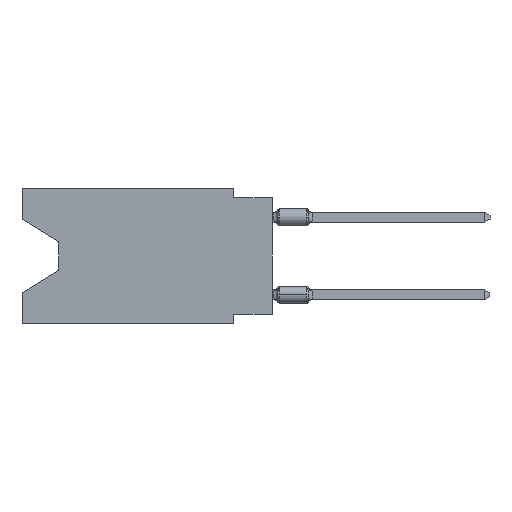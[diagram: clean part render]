
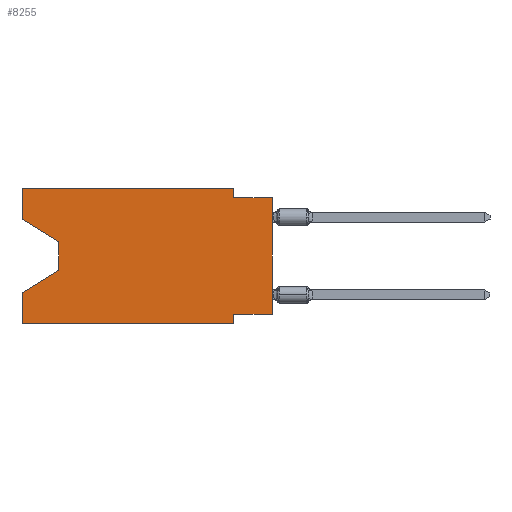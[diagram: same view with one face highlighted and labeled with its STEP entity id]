
A CAD part, left-side view. The second image highlights one B-rep face of the part: STEP entity #8255.
In plain terms, the highlighted planar face has unit normal (-1, 0, 0).
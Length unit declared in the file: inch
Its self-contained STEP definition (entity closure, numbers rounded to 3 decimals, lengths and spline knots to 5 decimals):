
#183 = CARTESIAN_POINT ( 'NONE',  ( 0., 0.645, 0. ) ) ;
#287 = EDGE_CURVE ( 'NONE', #10213, #3877, #16952, .T. ) ;
#308 = CARTESIAN_POINT ( 'NONE',  ( 0., 0.645, 0. ) ) ;
#857 = LINE ( 'NONE', #308, #16641 ) ;
#1285 = DIRECTION ( 'NONE',  ( 0., -1., 0. ) ) ;
#1613 = CARTESIAN_POINT ( 'NONE',  ( 0., 0.55, -0.212 ) ) ;
#1636 = EDGE_CURVE ( 'NONE', #25814, #21088, #18660, .T. ) ;
#1788 = CARTESIAN_POINT ( 'NONE',  ( 0., 0.645, -0.08025 ) ) ;
#1929 = DIRECTION ( 'NONE',  ( 0., -1., 0. ) ) ;
#2426 = DIRECTION ( 'NONE',  ( 0., 0., 1. ) ) ;
#3229 = CARTESIAN_POINT ( 'NONE',  ( 0., 0., -0.325 ) ) ;
#3236 = VECTOR ( 'NONE', #19499, 39.37008 ) ;
#3754 = EDGE_CURVE ( 'NONE', #13657, #24154, #13965, .T. ) ;
#3877 = VERTEX_POINT ( 'NONE', #27752 ) ;
#3882 = PLANE ( 'NONE',  #23036 ) ;
#4906 = EDGE_CURVE ( 'NONE', #6067, #7350, #11999, .T. ) ;
#4974 = DIRECTION ( 'NONE',  ( 0., 0., -1. ) ) ;
#5083 = VECTOR ( 'NONE', #4974, 39.37008 ) ;
#5327 = CARTESIAN_POINT ( 'NONE',  ( 0., 0.645, 0. ) ) ;
#6067 = VERTEX_POINT ( 'NONE', #19371 ) ;
#6144 = ORIENTED_EDGE ( 'NONE', *, *, #21571, .F. ) ;
#6408 = ORIENTED_EDGE ( 'NONE', *, *, #4906, .T. ) ;
#6532 = CARTESIAN_POINT ( 'NONE',  ( 0., 0.645, -0.26975 ) ) ;
#6679 = VECTOR ( 'NONE', #8355, 39.37008 ) ;
#6685 = EDGE_CURVE ( 'NONE', #6067, #21088, #857, .T. ) ;
#6865 = DIRECTION ( 'NONE',  ( 0., 0., 1. ) ) ;
#7350 = VERTEX_POINT ( 'NONE', #10551 ) ;
#8111 = DIRECTION ( 'NONE',  ( 1., 0., 0. ) ) ;
#8255 = ADVANCED_FACE ( 'NONE', ( #20650 ), #3882, .F. ) ;
#8355 = DIRECTION ( 'NONE',  ( 0., 1., 0. ) ) ;
#8492 = DIRECTION ( 'NONE',  ( 0., 0., -1. ) ) ;
#8881 = EDGE_CURVE ( 'NONE', #13657, #10913, #22809, .T. ) ;
#8960 = LINE ( 'NONE', #21652, #16801 ) ;
#9601 = CARTESIAN_POINT ( 'NONE',  ( 0., 0.645, -0.08025 ) ) ;
#10175 = CARTESIAN_POINT ( 'NONE',  ( 0., 0., -0.325 ) ) ;
#10199 = DIRECTION ( 'NONE',  ( 0., 0.855, -0.519 ) ) ;
#10213 = VERTEX_POINT ( 'NONE', #22694 ) ;
#10222 = CARTESIAN_POINT ( 'NONE',  ( 0., 0.645, 0. ) ) ;
#10230 = ORIENTED_EDGE ( 'NONE', *, *, #27822, .F. ) ;
#10551 = CARTESIAN_POINT ( 'NONE',  ( 0., 0.1, -0.35 ) ) ;
#10596 = ORIENTED_EDGE ( 'NONE', *, *, #13782, .T. ) ;
#10913 = VERTEX_POINT ( 'NONE', #17438 ) ;
#11261 = EDGE_CURVE ( 'NONE', #24154, #25814, #19210, .T. ) ;
#11999 = LINE ( 'NONE', #16370, #15288 ) ;
#12247 = VECTOR ( 'NONE', #26757, 39.37008 ) ;
#12577 = CARTESIAN_POINT ( 'NONE',  ( 0., 0.1, 0. ) ) ;
#13657 = VERTEX_POINT ( 'NONE', #1788 ) ;
#13782 = EDGE_CURVE ( 'NONE', #16031, #18413, #8960, .T. ) ;
#13953 = CARTESIAN_POINT ( 'NONE',  ( 0., 0.1, -0.325 ) ) ;
#13965 = LINE ( 'NONE', #9601, #26062 ) ;
#14239 = ORIENTED_EDGE ( 'NONE', *, *, #27090, .F. ) ;
#14951 = VECTOR ( 'NONE', #8492, 39.37008 ) ;
#15288 = VECTOR ( 'NONE', #1285, 39.37008 ) ;
#15967 = ORIENTED_EDGE ( 'NONE', *, *, #287, .F. ) ;
#16031 = VERTEX_POINT ( 'NONE', #3229 ) ;
#16094 = DIRECTION ( 'NONE',  ( 0., -0.855, -0.519 ) ) ;
#16370 = CARTESIAN_POINT ( 'NONE',  ( 0., 0.645, -0.35 ) ) ;
#16641 = VECTOR ( 'NONE', #2426, 39.37008 ) ;
#16756 = CARTESIAN_POINT ( 'NONE',  ( 0., 0.55, -0.138 ) ) ;
#16801 = VECTOR ( 'NONE', #6865, 39.37008 ) ;
#16952 = LINE ( 'NONE', #12577, #19095 ) ;
#17114 = EDGE_CURVE ( 'NONE', #10913, #10213, #23853, .T. ) ;
#17438 = CARTESIAN_POINT ( 'NONE',  ( 0., 0.645, 0. ) ) ;
#17806 = LINE ( 'NONE', #24274, #5083 ) ;
#18413 = VERTEX_POINT ( 'NONE', #23126 ) ;
#18660 = LINE ( 'NONE', #1613, #22263 ) ;
#19095 = VECTOR ( 'NONE', #27387, 39.37008 ) ;
#19210 = LINE ( 'NONE', #27151, #14951 ) ;
#19371 = CARTESIAN_POINT ( 'NONE',  ( 0., 0.645, -0.35 ) ) ;
#19499 = DIRECTION ( 'NONE',  ( 0., -1., 0. ) ) ;
#20038 = VERTEX_POINT ( 'NONE', #13953 ) ;
#20404 = ORIENTED_EDGE ( 'NONE', *, *, #3754, .T. ) ;
#20650 = FACE_OUTER_BOUND ( 'NONE', #23378, .T. ) ;
#21088 = VERTEX_POINT ( 'NONE', #6532 ) ;
#21236 = CARTESIAN_POINT ( 'NONE',  ( 0., 0., -0.025 ) ) ;
#21571 = EDGE_CURVE ( 'NONE', #20038, #7350, #17806, .T. ) ;
#21652 = CARTESIAN_POINT ( 'NONE',  ( 0., 0., 0. ) ) ;
#22263 = VECTOR ( 'NONE', #10199, 39.37008 ) ;
#22691 = ORIENTED_EDGE ( 'NONE', *, *, #11261, .T. ) ;
#22694 = CARTESIAN_POINT ( 'NONE',  ( 0., 0.1, 0. ) ) ;
#22722 = ORIENTED_EDGE ( 'NONE', *, *, #6685, .F. ) ;
#22809 = LINE ( 'NONE', #5327, #12247 ) ;
#23036 = AXIS2_PLACEMENT_3D ( 'NONE', #10222, #8111, #27417 ) ;
#23126 = CARTESIAN_POINT ( 'NONE',  ( 0., 0., -0.025 ) ) ;
#23378 = EDGE_LOOP ( 'NONE', ( #20404, #22691, #23581, #22722, #6408, #6144, #10230, #10596, #14239, #15967, #27141, #24167 ) ) ;
#23581 = ORIENTED_EDGE ( 'NONE', *, *, #1636, .T. ) ;
#23628 = LINE ( 'NONE', #21236, #26887 ) ;
#23853 = LINE ( 'NONE', #183, #3236 ) ;
#24154 = VERTEX_POINT ( 'NONE', #16756 ) ;
#24167 = ORIENTED_EDGE ( 'NONE', *, *, #8881, .F. ) ;
#24274 = CARTESIAN_POINT ( 'NONE',  ( 0., 0.1, -0.35 ) ) ;
#25814 = VERTEX_POINT ( 'NONE', #27432 ) ;
#26062 = VECTOR ( 'NONE', #16094, 39.37008 ) ;
#26757 = DIRECTION ( 'NONE',  ( 0., 0., 1. ) ) ;
#26887 = VECTOR ( 'NONE', #1929, 39.37008 ) ;
#27090 = EDGE_CURVE ( 'NONE', #3877, #18413, #23628, .T. ) ;
#27141 = ORIENTED_EDGE ( 'NONE', *, *, #17114, .F. ) ;
#27151 = CARTESIAN_POINT ( 'NONE',  ( 0., 0.55, -0.138 ) ) ;
#27387 = DIRECTION ( 'NONE',  ( 0., 0., -1. ) ) ;
#27417 = DIRECTION ( 'NONE',  ( 0., 0., -1. ) ) ;
#27432 = CARTESIAN_POINT ( 'NONE',  ( 0., 0.55, -0.212 ) ) ;
#27657 = LINE ( 'NONE', #10175, #6679 ) ;
#27752 = CARTESIAN_POINT ( 'NONE',  ( 0., 0.1, -0.025 ) ) ;
#27822 = EDGE_CURVE ( 'NONE', #16031, #20038, #27657, .T. ) ;
